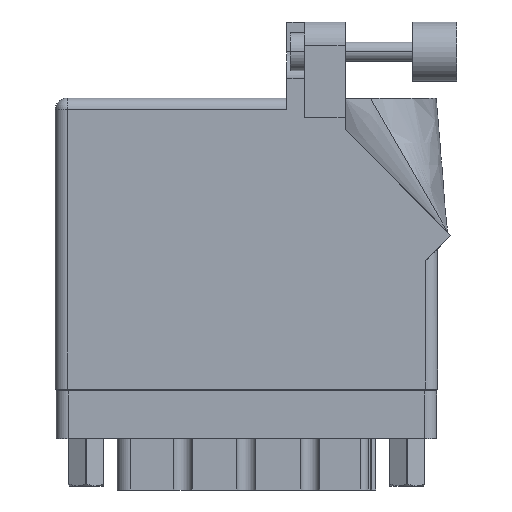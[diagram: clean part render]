
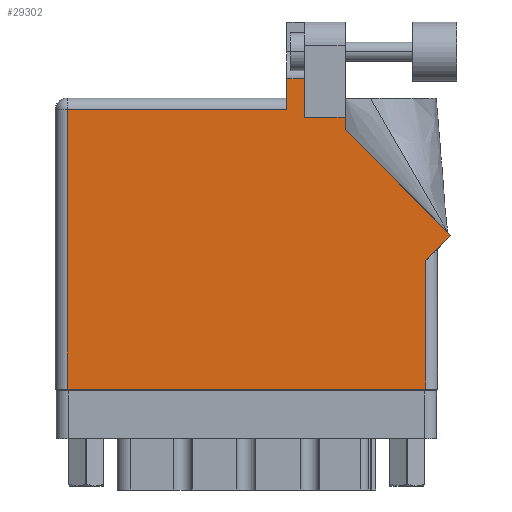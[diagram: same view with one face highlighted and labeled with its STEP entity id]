
A CAD part, front view. The second image highlights one B-rep face of the part: STEP entity #29302.
In plain terms, the highlighted face is planar.
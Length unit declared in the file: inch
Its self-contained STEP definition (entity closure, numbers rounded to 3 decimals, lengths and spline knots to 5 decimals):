
#1051 = LINE ( 'NONE', #36141, #31949 ) ;
#1555 = DIRECTION ( 'NONE',  ( -1., 0., 0. ) ) ;
#2108 = CARTESIAN_POINT ( 'NONE',  ( 1.948, 0.675, 0. ) ) ;
#2314 = VECTOR ( 'NONE', #23915, 39.37008 ) ;
#2660 = DIRECTION ( 'NONE',  ( -1., 0., 0. ) ) ;
#3360 = ORIENTED_EDGE ( 'NONE', *, *, #48258, .T. ) ;
#3706 = VECTOR ( 'NONE', #17339, 39.37008 ) ;
#4573 = EDGE_LOOP ( 'NONE', ( #32130, #4710, #5840, #3360, #6292, #15128, #30742, #29979, #23922, #37005, #38499 ) ) ;
#4710 = ORIENTED_EDGE ( 'NONE', *, *, #4837, .T. ) ;
#4837 = EDGE_CURVE ( 'NONE', #28377, #35917, #26069, .T. ) ;
#4843 = CARTESIAN_POINT ( 'NONE',  ( 0., 0., 0. ) ) ;
#5840 = ORIENTED_EDGE ( 'NONE', *, *, #27560, .T. ) ;
#6292 = ORIENTED_EDGE ( 'NONE', *, *, #42546, .T. ) ;
#6490 = LINE ( 'NONE', #29106, #43035 ) ;
#6544 = VECTOR ( 'NONE', #34075, 39.37008 ) ;
#6762 = CARTESIAN_POINT ( 'NONE',  ( 1.64177, 1.6315, 0. ) ) ;
#6872 = CARTESIAN_POINT ( 'NONE',  ( 1.311, 1.6315, 0. ) ) ;
#7938 = AXIS2_PLACEMENT_3D ( 'NONE', #32330, #47126, #43056 ) ;
#8538 = CARTESIAN_POINT ( 'NONE',  ( 1.217, 1.468, 0. ) ) ;
#9423 = LINE ( 'NONE', #28989, #37770 ) ;
#10221 = VERTEX_POINT ( 'NONE', #8538 ) ;
#10792 = VECTOR ( 'NONE', #49231, 39.37008 ) ;
#11293 = VERTEX_POINT ( 'NONE', #33804 ) ;
#12731 = DIRECTION ( 'NONE',  ( 0., 1., 0. ) ) ;
#12992 = CARTESIAN_POINT ( 'NONE',  ( 1.311, 1.43, 0. ) ) ;
#13720 = CARTESIAN_POINT ( 'NONE',  ( 1.948, 0., 0. ) ) ;
#15128 = ORIENTED_EDGE ( 'NONE', *, *, #17165, .T. ) ;
#15486 = CARTESIAN_POINT ( 'NONE',  ( 1.217, 1.53, 0. ) ) ;
#16802 = PLANE ( 'NONE',  #7938 ) ;
#17165 = EDGE_CURVE ( 'NONE', #24094, #21557, #28228, .T. ) ;
#17339 = DIRECTION ( 'NONE',  ( 0., 1., 0. ) ) ;
#17488 = VERTEX_POINT ( 'NONE', #25478 ) ;
#19317 = CARTESIAN_POINT ( 'NONE',  ( 2.08071, 0.80771, 0. ) ) ;
#19494 = CARTESIAN_POINT ( 'NONE',  ( 0.062, 0., 0. ) ) ;
#21106 = VECTOR ( 'NONE', #34832, 39.37008 ) ;
#21545 = CARTESIAN_POINT ( 'NONE',  ( 0.062, 1.468, 0. ) ) ;
#21557 = VERTEX_POINT ( 'NONE', #13720 ) ;
#23915 = DIRECTION ( 'NONE',  ( 1., 0., 0. ) ) ;
#23922 = ORIENTED_EDGE ( 'NONE', *, *, #37474, .T. ) ;
#24094 = VERTEX_POINT ( 'NONE', #19494 ) ;
#25478 = CARTESIAN_POINT ( 'NONE',  ( 1.524, 1.43, 0. ) ) ;
#26069 = LINE ( 'NONE', #6762, #46400 ) ;
#26426 = LINE ( 'NONE', #42729, #6544 ) ;
#26860 = VERTEX_POINT ( 'NONE', #21545 ) ;
#27147 = EDGE_CURVE ( 'NONE', #31096, #28377, #32621, .T. ) ;
#27419 = DIRECTION ( 'NONE',  ( 0., -1., 0. ) ) ;
#27560 = EDGE_CURVE ( 'NONE', #35917, #10221, #46042, .T. ) ;
#27875 = CARTESIAN_POINT ( 'NONE',  ( 2.08071, 0.80771, 0. ) ) ;
#28228 = LINE ( 'NONE', #4843, #2314 ) ;
#28377 = VERTEX_POINT ( 'NONE', #6872 ) ;
#28989 = CARTESIAN_POINT ( 'NONE',  ( 1.524, 1.36442, 0. ) ) ;
#29106 = CARTESIAN_POINT ( 'NONE',  ( 1.524, 1.43, 0. ) ) ;
#29302 = ADVANCED_FACE ( 'NONE', ( #31589 ), #16802, .F. ) ;
#29979 = ORIENTED_EDGE ( 'NONE', *, *, #37394, .T. ) ;
#30311 = VECTOR ( 'NONE', #31321, 39.37008 ) ;
#30742 = ORIENTED_EDGE ( 'NONE', *, *, #46542, .T. ) ;
#31096 = VERTEX_POINT ( 'NONE', #12992 ) ;
#31321 = DIRECTION ( 'NONE',  ( 0., 1., 0. ) ) ;
#31589 = FACE_OUTER_BOUND ( 'NONE', #4573, .T. ) ;
#31949 = VECTOR ( 'NONE', #1555, 39.37008 ) ;
#32130 = ORIENTED_EDGE ( 'NONE', *, *, #27147, .T. ) ;
#32330 = CARTESIAN_POINT ( 'NONE',  ( 0., 1.53, 0. ) ) ;
#32621 = LINE ( 'NONE', #40773, #3706 ) ;
#33804 = CARTESIAN_POINT ( 'NONE',  ( 1.524, 1.36442, 0. ) ) ;
#33928 = CARTESIAN_POINT ( 'NONE',  ( 0.062, 0., 0. ) ) ;
#34075 = DIRECTION ( 'NONE',  ( 0.707, 0.707, 0. ) ) ;
#34832 = DIRECTION ( 'NONE',  ( -0.707, 0.707, 0. ) ) ;
#35917 = VERTEX_POINT ( 'NONE', #39400 ) ;
#36141 = CARTESIAN_POINT ( 'NONE',  ( 0., 1.468, 0. ) ) ;
#36401 = EDGE_CURVE ( 'NONE', #17488, #31096, #6490, .T. ) ;
#37005 = ORIENTED_EDGE ( 'NONE', *, *, #49945, .T. ) ;
#37394 = EDGE_CURVE ( 'NONE', #49470, #39935, #26426, .T. ) ;
#37474 = EDGE_CURVE ( 'NONE', #39935, #11293, #50129, .T. ) ;
#37760 = LINE ( 'NONE', #33928, #10792 ) ;
#37770 = VECTOR ( 'NONE', #12731, 39.37008 ) ;
#38047 = DIRECTION ( 'NONE',  ( -1., 0., 0. ) ) ;
#38454 = LINE ( 'NONE', #46355, #30311 ) ;
#38499 = ORIENTED_EDGE ( 'NONE', *, *, #36401, .T. ) ;
#39400 = CARTESIAN_POINT ( 'NONE',  ( 1.217, 1.6315, 0. ) ) ;
#39526 = VECTOR ( 'NONE', #27419, 39.37008 ) ;
#39935 = VERTEX_POINT ( 'NONE', #27875 ) ;
#40773 = CARTESIAN_POINT ( 'NONE',  ( 1.311, 1.43, 0. ) ) ;
#42546 = EDGE_CURVE ( 'NONE', #26860, #24094, #37760, .T. ) ;
#42729 = CARTESIAN_POINT ( 'NONE',  ( 2.01, 0.737, 0. ) ) ;
#43035 = VECTOR ( 'NONE', #2660, 39.37008 ) ;
#43056 = DIRECTION ( 'NONE',  ( -1., 0., 0. ) ) ;
#46042 = LINE ( 'NONE', #15486, #39526 ) ;
#46355 = CARTESIAN_POINT ( 'NONE',  ( 1.948, 0.737, 0. ) ) ;
#46400 = VECTOR ( 'NONE', #38047, 39.37008 ) ;
#46542 = EDGE_CURVE ( 'NONE', #21557, #49470, #38454, .T. ) ;
#47126 = DIRECTION ( 'NONE',  ( 0., 0., -1. ) ) ;
#48258 = EDGE_CURVE ( 'NONE', #10221, #26860, #1051, .T. ) ;
#49231 = DIRECTION ( 'NONE',  ( 0., -1., 0. ) ) ;
#49470 = VERTEX_POINT ( 'NONE', #2108 ) ;
#49945 = EDGE_CURVE ( 'NONE', #11293, #17488, #9423, .T. ) ;
#50129 = LINE ( 'NONE', #19317, #21106 ) ;
